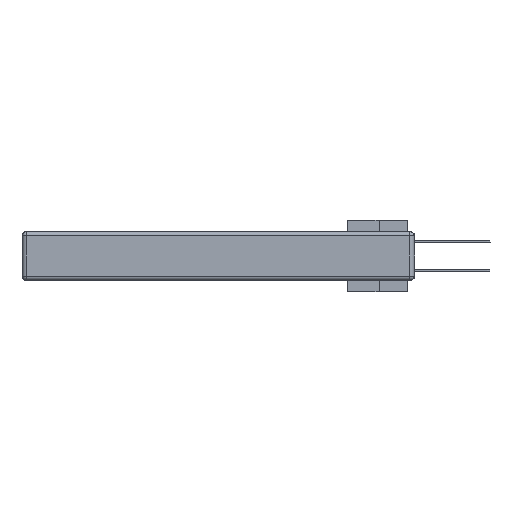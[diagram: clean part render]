
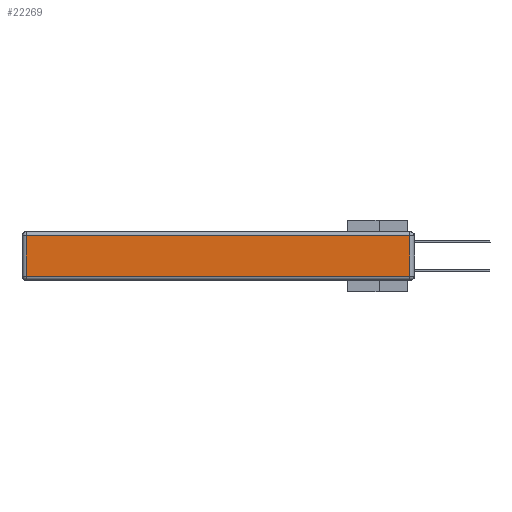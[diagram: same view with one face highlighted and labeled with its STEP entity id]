
A CAD part, left-side view. The second image highlights one B-rep face of the part: STEP entity #22269.
In plain terms, the highlighted planar face has unit normal (-1, 0, 0).
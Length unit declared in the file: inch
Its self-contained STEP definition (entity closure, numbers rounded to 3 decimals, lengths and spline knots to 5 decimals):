
#316 = DIRECTION ( 'NONE',  ( -1., 0., 0. ) ) ;
#687 = ORIENTED_EDGE ( 'NONE', *, *, #16965, .T. ) ;
#1737 = EDGE_CURVE ( 'NONE', #8078, #24757, #11986, .T. ) ;
#1868 = DIRECTION ( 'NONE',  ( 0., 0., -1. ) ) ;
#1964 = EDGE_LOOP ( 'NONE', ( #6180, #27471, #687, #25645 ) ) ;
#4667 = AXIS2_PLACEMENT_3D ( 'NONE', #26859, #316, #18771 ) ;
#6180 = ORIENTED_EDGE ( 'NONE', *, *, #1737, .T. ) ;
#7243 = DIRECTION ( 'NONE',  ( 0., 0., 1. ) ) ;
#8078 = VERTEX_POINT ( 'NONE', #24452 ) ;
#9279 = CARTESIAN_POINT ( 'NONE',  ( 0., 2.75, -0.03 ) ) ;
#9823 = CARTESIAN_POINT ( 'NONE',  ( 0., 2.72, -0.03 ) ) ;
#11986 = LINE ( 'NONE', #29531, #20371 ) ;
#12739 = EDGE_CURVE ( 'NONE', #28117, #8078, #17993, .T. ) ;
#12747 = LINE ( 'NONE', #9279, #29155 ) ;
#15013 = CARTESIAN_POINT ( 'NONE',  ( 0., 2.72, -0.343 ) ) ;
#16965 = EDGE_CURVE ( 'NONE', #17673, #28117, #12747, .T. ) ;
#17673 = VERTEX_POINT ( 'NONE', #25470 ) ;
#17993 = LINE ( 'NONE', #15013, #21734 ) ;
#18771 = DIRECTION ( 'NONE',  ( 0., 0., 1. ) ) ;
#19220 = CARTESIAN_POINT ( 'NONE',  ( 0., 0.03, -0.313 ) ) ;
#20255 = FACE_OUTER_BOUND ( 'NONE', #1964, .T. ) ;
#20364 = LINE ( 'NONE', #23799, #30417 ) ;
#20371 = VECTOR ( 'NONE', #27080, 39.37008 ) ;
#21734 = VECTOR ( 'NONE', #1868, 39.37008 ) ;
#22269 = ADVANCED_FACE ( 'NONE', ( #20255 ), #29897, .T. ) ;
#23799 = CARTESIAN_POINT ( 'NONE',  ( 0., 0.03, -0.343 ) ) ;
#24452 = CARTESIAN_POINT ( 'NONE',  ( 0., 2.72, -0.313 ) ) ;
#24757 = VERTEX_POINT ( 'NONE', #19220 ) ;
#25470 = CARTESIAN_POINT ( 'NONE',  ( 0., 0.03, -0.03 ) ) ;
#25645 = ORIENTED_EDGE ( 'NONE', *, *, #12739, .T. ) ;
#26859 = CARTESIAN_POINT ( 'NONE',  ( 0., 0., -0.343 ) ) ;
#27080 = DIRECTION ( 'NONE',  ( 0., -1., 0. ) ) ;
#27471 = ORIENTED_EDGE ( 'NONE', *, *, #28250, .T. ) ;
#28117 = VERTEX_POINT ( 'NONE', #9823 ) ;
#28250 = EDGE_CURVE ( 'NONE', #24757, #17673, #20364, .T. ) ;
#28342 = DIRECTION ( 'NONE',  ( 0., 1., 0. ) ) ;
#29155 = VECTOR ( 'NONE', #28342, 39.37008 ) ;
#29531 = CARTESIAN_POINT ( 'NONE',  ( 0., 0., -0.313 ) ) ;
#29897 = PLANE ( 'NONE',  #4667 ) ;
#30417 = VECTOR ( 'NONE', #7243, 39.37008 ) ;
